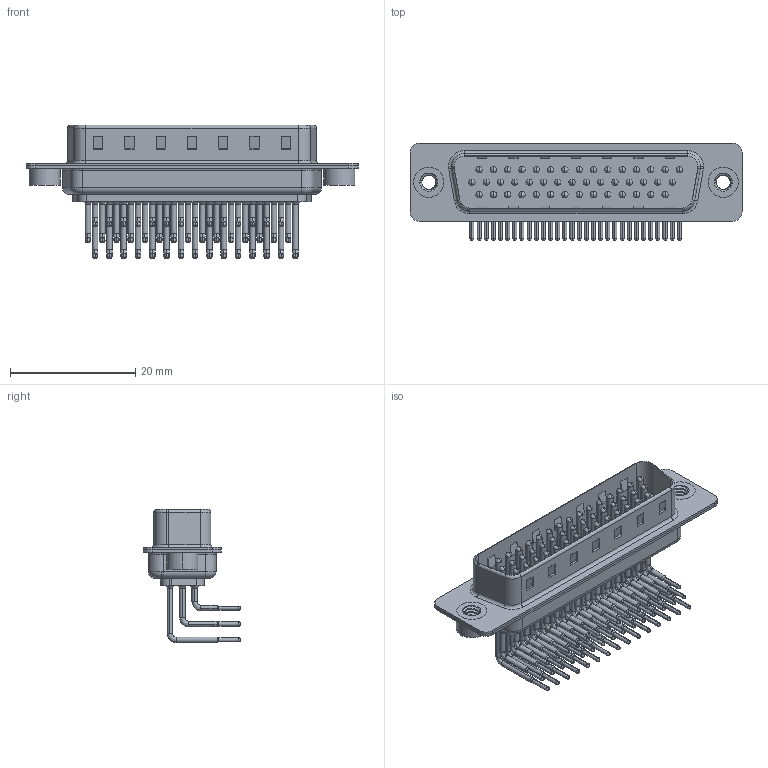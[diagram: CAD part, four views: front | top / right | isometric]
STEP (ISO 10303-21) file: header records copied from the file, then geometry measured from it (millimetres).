
FILE_DESCRIPTION (( 'STEP AP203' ), '1' );
FILE_NAME ('633-M44-663-WN2.STEP', '2018-09-28T01:50:53', ( '' ), ( '' ), 'SwSTEP 2.0', 'SolidWorks 2016', '' );
FILE_SCHEMA (( 'CONFIG_CONTROL_DESIGN' ));
Length unit declared in the file: millimetre
Products named in the file (8): 633M Contact Row 3; 633M 4-40 Threaded Rivet; 633-M44-663-WN2; 633M Housing_44 Contacts; 633M Shell Front_44 Contacts; 633M Shell Rear_44 Contacts; 633M Contact Row 1; 633M Contact Row 2
Assembly tree (49 placements, depth 2):
  633-M44-663-WN2
    633M Housing_44 Contacts
    633M Shell Front_44 Contacts
    633M Shell Rear_44 Contacts
    633M Contact Row 1  x15
    633M Contact Row 2  x15
    633M Contact Row 3  x14
    633M 4-40 Threaded Rivet  x2
Bounding box: 53.05 x 15.6 x 21.32 mm (x, y, z)
Volume: 3136.1 mm3; surface area: 10056.5 mm2
Topology: 49 solids, 49 shells, 5216 faces, 14629 edges, 9522 vertices
Faces by surface type: plane 2987, cylinder 1721, bspline 270, cone 182, torus 56
Entity records: 34422 total; most frequent: CARTESIAN_POINT 7074, DIRECTION 5593, ORIENTED_EDGE 5070, EDGE_CURVE 2535, AXIS2_PLACEMENT_3D 2075, VERTEX_POINT 1651, VECTOR 1443, LINE 1443
